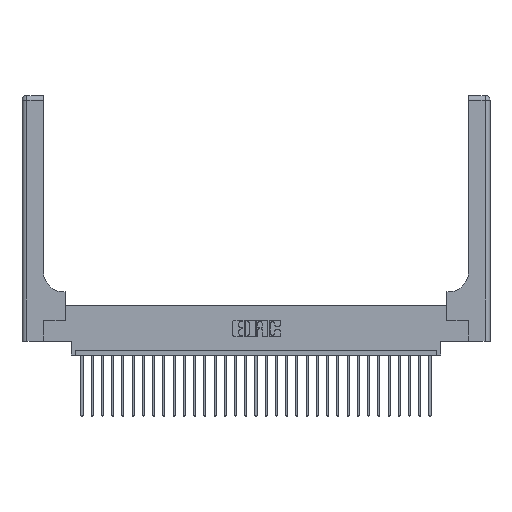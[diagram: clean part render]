
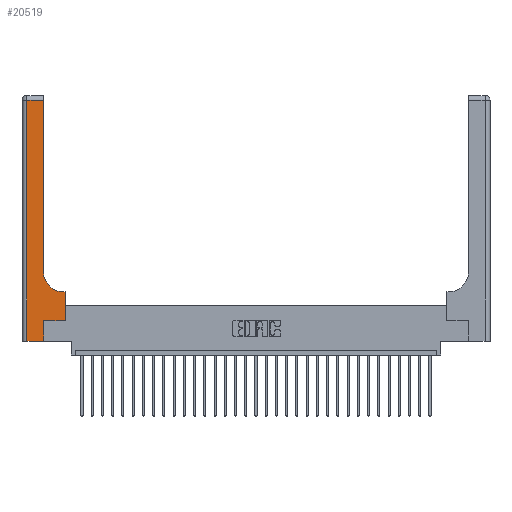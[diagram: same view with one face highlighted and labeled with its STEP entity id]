
A CAD part, top view. The second image highlights one B-rep face of the part: STEP entity #20519.
In plain terms, the highlighted planar face has unit normal (0, 0, 1).
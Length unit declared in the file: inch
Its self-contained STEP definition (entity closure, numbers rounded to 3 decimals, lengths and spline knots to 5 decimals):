
#271 = DIRECTION ( 'NONE',  ( 0., 1., 0. ) ) ;
#874 = ORIENTED_EDGE ( 'NONE', *, *, #19160, .T. ) ;
#1747 = VECTOR ( 'NONE', #271, 39.37008 ) ;
#1841 = CARTESIAN_POINT ( 'NONE',  ( 0.528, 0.6, 0.37 ) ) ;
#2215 = VERTEX_POINT ( 'NONE', #17439 ) ;
#2549 = CARTESIAN_POINT ( 'NONE',  ( 0.26, 0.85, 0.37 ) ) ;
#3079 = VERTEX_POINT ( 'NONE', #26083 ) ;
#3120 = EDGE_CURVE ( 'NONE', #26541, #2215, #26672, .T. ) ;
#3373 = ORIENTED_EDGE ( 'NONE', *, *, #21549, .T. ) ;
#3921 = VECTOR ( 'NONE', #27172, 39.37008 ) ;
#4647 = CARTESIAN_POINT ( 'NONE',  ( 0.265, 0.25, 0.37 ) ) ;
#4866 = ORIENTED_EDGE ( 'NONE', *, *, #3120, .T. ) ;
#4970 = CARTESIAN_POINT ( 'NONE',  ( 0.26, 2.94, 0.37 ) ) ;
#5097 = VECTOR ( 'NONE', #27823, 39.37008 ) ;
#5211 = EDGE_CURVE ( 'NONE', #2215, #18349, #22163, .T. ) ;
#5237 = CIRCLE ( 'NONE', #12684, 0.25 ) ;
#5776 = VECTOR ( 'NONE', #16625, 39.37008 ) ;
#6242 = CARTESIAN_POINT ( 'NONE',  ( 0.26, 3., 0.37 ) ) ;
#6249 = PLANE ( 'NONE',  #25478 ) ;
#6595 = ORIENTED_EDGE ( 'NONE', *, *, #11427, .T. ) ;
#7794 = CARTESIAN_POINT ( 'NONE',  ( 0.06, 3., 0.37 ) ) ;
#7820 = LINE ( 'NONE', #23232, #5097 ) ;
#7970 = VERTEX_POINT ( 'NONE', #21092 ) ;
#8132 = EDGE_LOOP ( 'NONE', ( #25690, #16153, #19219, #874, #16521, #4866, #26032, #3373, #6595 ) ) ;
#8394 = DIRECTION ( 'NONE',  ( -1., 0., 0. ) ) ;
#8655 = CARTESIAN_POINT ( 'NONE',  ( 0.06, 2.94, 0.37 ) ) ;
#9280 = DIRECTION ( 'NONE',  ( 1., 0., 0. ) ) ;
#10404 = VECTOR ( 'NONE', #9280, 39.37008 ) ;
#11126 = CARTESIAN_POINT ( 'NONE',  ( 0.51, 0.6, 0.37 ) ) ;
#11427 = EDGE_CURVE ( 'NONE', #17636, #15568, #5237, .T. ) ;
#11794 = LINE ( 'NONE', #20566, #3921 ) ;
#12684 = AXIS2_PLACEMENT_3D ( 'NONE', #25893, #23593, #14852 ) ;
#12783 = VECTOR ( 'NONE', #8394, 39.37008 ) ;
#12904 = LINE ( 'NONE', #6242, #28370 ) ;
#13962 = EDGE_CURVE ( 'NONE', #15538, #20838, #14892, .T. ) ;
#14366 = EDGE_CURVE ( 'NONE', #3079, #26541, #18340, .T. ) ;
#14852 = DIRECTION ( 'NONE',  ( 1., 0., 0. ) ) ;
#14892 = LINE ( 'NONE', #17474, #12783 ) ;
#15538 = VERTEX_POINT ( 'NONE', #4970 ) ;
#15568 = VERTEX_POINT ( 'NONE', #2549 ) ;
#16153 = ORIENTED_EDGE ( 'NONE', *, *, #13962, .T. ) ;
#16201 = DIRECTION ( 'NONE',  ( 0., 1., 0. ) ) ;
#16521 = ORIENTED_EDGE ( 'NONE', *, *, #14366, .T. ) ;
#16625 = DIRECTION ( 'NONE',  ( 0., -1., 0. ) ) ;
#17374 = CARTESIAN_POINT ( 'NONE',  ( 0., 3., 0.37 ) ) ;
#17438 = CARTESIAN_POINT ( 'NONE',  ( 0.265, 0.25, 0.37 ) ) ;
#17439 = CARTESIAN_POINT ( 'NONE',  ( 0.528, 0.25, 0.37 ) ) ;
#17474 = CARTESIAN_POINT ( 'NONE',  ( 0., 2.94, 0.37 ) ) ;
#17636 = VERTEX_POINT ( 'NONE', #11126 ) ;
#18340 = LINE ( 'NONE', #27094, #24758 ) ;
#18349 = VERTEX_POINT ( 'NONE', #1841 ) ;
#18974 = FACE_OUTER_BOUND ( 'NONE', #8132, .T. ) ;
#19160 = EDGE_CURVE ( 'NONE', #7970, #3079, #7820, .T. ) ;
#19219 = ORIENTED_EDGE ( 'NONE', *, *, #22845, .T. ) ;
#19992 = CARTESIAN_POINT ( 'NONE',  ( 0.528, 0.25, 0.37 ) ) ;
#20519 = ADVANCED_FACE ( 'NONE', ( #18974 ), #6249, .F. ) ;
#20566 = CARTESIAN_POINT ( 'NONE',  ( 0.26, 0.6, 0.37 ) ) ;
#20838 = VERTEX_POINT ( 'NONE', #8655 ) ;
#21092 = CARTESIAN_POINT ( 'NONE',  ( 0.06, 0., 0.37 ) ) ;
#21549 = EDGE_CURVE ( 'NONE', #18349, #17636, #11794, .T. ) ;
#22163 = LINE ( 'NONE', #19992, #1747 ) ;
#22845 = EDGE_CURVE ( 'NONE', #20838, #7970, #27517, .T. ) ;
#23232 = CARTESIAN_POINT ( 'NONE',  ( 0., 0., 0.37 ) ) ;
#23593 = DIRECTION ( 'NONE',  ( 0., 0., -1. ) ) ;
#24758 = VECTOR ( 'NONE', #16201, 39.37008 ) ;
#25478 = AXIS2_PLACEMENT_3D ( 'NONE', #17374, #25847, #27860 ) ;
#25690 = ORIENTED_EDGE ( 'NONE', *, *, #26743, .T. ) ;
#25840 = DIRECTION ( 'NONE',  ( 0., 1., 0. ) ) ;
#25847 = DIRECTION ( 'NONE',  ( 0., 0., -1. ) ) ;
#25893 = CARTESIAN_POINT ( 'NONE',  ( 0.51, 0.85, 0.37 ) ) ;
#26032 = ORIENTED_EDGE ( 'NONE', *, *, #5211, .T. ) ;
#26083 = CARTESIAN_POINT ( 'NONE',  ( 0.265, 0., 0.37 ) ) ;
#26541 = VERTEX_POINT ( 'NONE', #17438 ) ;
#26672 = LINE ( 'NONE', #4647, #10404 ) ;
#26743 = EDGE_CURVE ( 'NONE', #15568, #15538, #12904, .T. ) ;
#27094 = CARTESIAN_POINT ( 'NONE',  ( 0.265, 0., 0.37 ) ) ;
#27172 = DIRECTION ( 'NONE',  ( -1., 0., 0. ) ) ;
#27517 = LINE ( 'NONE', #7794, #5776 ) ;
#27823 = DIRECTION ( 'NONE',  ( 1., 0., 0. ) ) ;
#27860 = DIRECTION ( 'NONE',  ( -1., 0., 0. ) ) ;
#28370 = VECTOR ( 'NONE', #25840, 39.37008 ) ;
